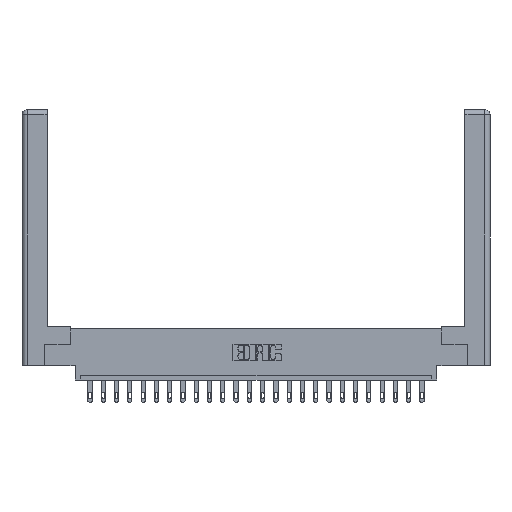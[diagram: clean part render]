
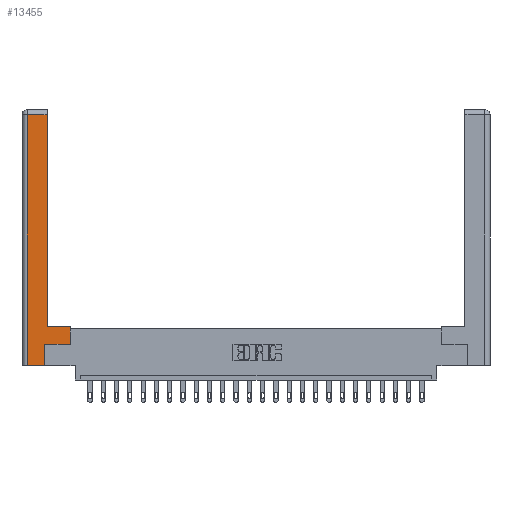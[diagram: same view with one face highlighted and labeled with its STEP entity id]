
A CAD part, top view. The second image highlights one B-rep face of the part: STEP entity #13455.
In plain terms, the highlighted planar face has unit normal (0, 0, 1).
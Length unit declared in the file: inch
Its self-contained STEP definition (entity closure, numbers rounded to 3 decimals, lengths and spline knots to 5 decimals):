
#277 = LINE ( 'NONE', #21835, #7022 ) ;
#325 = FACE_OUTER_BOUND ( 'NONE', #15290, .T. ) ;
#522 = DIRECTION ( 'NONE',  ( 0., 1., 0. ) ) ;
#596 = DIRECTION ( 'NONE',  ( 0., 1., 0. ) ) ;
#661 = CARTESIAN_POINT ( 'NONE',  ( 0.565, 0.245, 0. ) ) ;
#888 = LINE ( 'NONE', #15377, #1769 ) ;
#1147 = DIRECTION ( 'NONE',  ( 1., 0., 0. ) ) ;
#1509 = LINE ( 'NONE', #18224, #20459 ) ;
#1680 = CARTESIAN_POINT ( 'NONE',  ( 0.0615, 2.94, 0. ) ) ;
#1769 = VECTOR ( 'NONE', #596, 39.37008 ) ;
#2037 = VERTEX_POINT ( 'NONE', #8195 ) ;
#2116 = VERTEX_POINT ( 'NONE', #19569 ) ;
#2387 = CARTESIAN_POINT ( 'NONE',  ( 0., 0., 0. ) ) ;
#2503 = CARTESIAN_POINT ( 'NONE',  ( 0.0615, 0., 0. ) ) ;
#2942 = VERTEX_POINT ( 'NONE', #19640 ) ;
#3705 = CARTESIAN_POINT ( 'NONE',  ( 0.0615, 0., 0. ) ) ;
#4223 = VECTOR ( 'NONE', #19175, 39.37008 ) ;
#4243 = DIRECTION ( 'NONE',  ( -1., 0., 0. ) ) ;
#4441 = CARTESIAN_POINT ( 'NONE',  ( 0.265, 0.245, 0. ) ) ;
#4961 = ORIENTED_EDGE ( 'NONE', *, *, #5409, .T. ) ;
#5409 = EDGE_CURVE ( 'NONE', #19772, #12325, #12663, .T. ) ;
#5655 = LINE ( 'NONE', #7603, #10003 ) ;
#6063 = VERTEX_POINT ( 'NONE', #1680 ) ;
#6613 = ORIENTED_EDGE ( 'NONE', *, *, #9593, .T. ) ;
#7022 = VECTOR ( 'NONE', #16314, 39.37008 ) ;
#7137 = VECTOR ( 'NONE', #1147, 39.37008 ) ;
#7603 = CARTESIAN_POINT ( 'NONE',  ( 0.265, 0., 0. ) ) ;
#7919 = EDGE_CURVE ( 'NONE', #2116, #6063, #16134, .T. ) ;
#8195 = CARTESIAN_POINT ( 'NONE',  ( 0.265, 0., 0. ) ) ;
#8291 = CARTESIAN_POINT ( 'NONE',  ( 0.295, 0.45, 0. ) ) ;
#8330 = DIRECTION ( 'NONE',  ( 0., 0., -1. ) ) ;
#8448 = ORIENTED_EDGE ( 'NONE', *, *, #14976, .T. ) ;
#8980 = DIRECTION ( 'NONE',  ( 0., 1., 0. ) ) ;
#8997 = VECTOR ( 'NONE', #522, 39.37008 ) ;
#9018 = EDGE_CURVE ( 'NONE', #22821, #2116, #1509, .T. ) ;
#9593 = EDGE_CURVE ( 'NONE', #2037, #19772, #888, .T. ) ;
#9749 = CARTESIAN_POINT ( 'NONE',  ( 0.565, 0.45, 0. ) ) ;
#9960 = DIRECTION ( 'NONE',  ( -1., 0., 0. ) ) ;
#10003 = VECTOR ( 'NONE', #24081, 39.37008 ) ;
#11243 = LINE ( 'NONE', #2503, #4223 ) ;
#11821 = VERTEX_POINT ( 'NONE', #3705 ) ;
#12325 = VERTEX_POINT ( 'NONE', #661 ) ;
#12663 = LINE ( 'NONE', #23484, #7137 ) ;
#13455 = ADVANCED_FACE ( 'NONE', ( #325 ), #19466, .F. ) ;
#13936 = LINE ( 'NONE', #9749, #8997 ) ;
#14976 = EDGE_CURVE ( 'NONE', #2942, #22821, #277, .T. ) ;
#15116 = ORIENTED_EDGE ( 'NONE', *, *, #20291, .T. ) ;
#15290 = EDGE_LOOP ( 'NONE', ( #21560, #22012, #15462, #15116, #6613, #4961, #21455, #8448 ) ) ;
#15377 = CARTESIAN_POINT ( 'NONE',  ( 0.265, 0.245, 0. ) ) ;
#15462 = ORIENTED_EDGE ( 'NONE', *, *, #22861, .T. ) ;
#15673 = CARTESIAN_POINT ( 'NONE',  ( 0.0615, 2.94, 0. ) ) ;
#16134 = LINE ( 'NONE', #15673, #17880 ) ;
#16314 = DIRECTION ( 'NONE',  ( -1., 0., 0. ) ) ;
#17487 = AXIS2_PLACEMENT_3D ( 'NONE', #2387, #8330, #4243 ) ;
#17536 = EDGE_CURVE ( 'NONE', #12325, #2942, #13936, .T. ) ;
#17880 = VECTOR ( 'NONE', #9960, 39.37008 ) ;
#18224 = CARTESIAN_POINT ( 'NONE',  ( 0.295, 3., 0. ) ) ;
#19175 = DIRECTION ( 'NONE',  ( 0., -1., 0. ) ) ;
#19466 = PLANE ( 'NONE',  #17487 ) ;
#19569 = CARTESIAN_POINT ( 'NONE',  ( 0.295, 2.94, 0. ) ) ;
#19640 = CARTESIAN_POINT ( 'NONE',  ( 0.565, 0.45, 0. ) ) ;
#19772 = VERTEX_POINT ( 'NONE', #4441 ) ;
#20291 = EDGE_CURVE ( 'NONE', #11821, #2037, #5655, .T. ) ;
#20459 = VECTOR ( 'NONE', #8980, 39.37008 ) ;
#21455 = ORIENTED_EDGE ( 'NONE', *, *, #17536, .T. ) ;
#21560 = ORIENTED_EDGE ( 'NONE', *, *, #9018, .T. ) ;
#21835 = CARTESIAN_POINT ( 'NONE',  ( 0.295, 0.45, 0. ) ) ;
#22012 = ORIENTED_EDGE ( 'NONE', *, *, #7919, .T. ) ;
#22821 = VERTEX_POINT ( 'NONE', #8291 ) ;
#22861 = EDGE_CURVE ( 'NONE', #6063, #11821, #11243, .T. ) ;
#23484 = CARTESIAN_POINT ( 'NONE',  ( 0.565, 0.245, 0. ) ) ;
#24081 = DIRECTION ( 'NONE',  ( 1., 0., 0. ) ) ;
